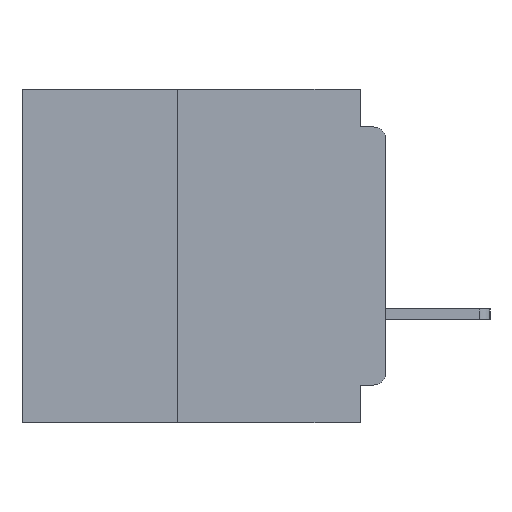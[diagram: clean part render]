
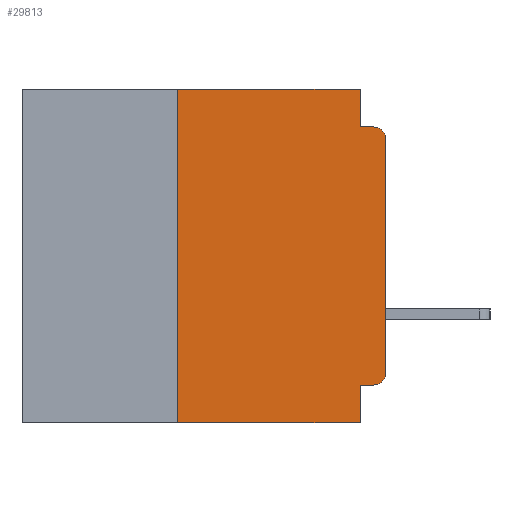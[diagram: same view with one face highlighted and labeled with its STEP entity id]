
A CAD part, left-side view. The second image highlights one B-rep face of the part: STEP entity #29813.
In plain terms, the highlighted planar face has unit normal (-1, 0, 0).
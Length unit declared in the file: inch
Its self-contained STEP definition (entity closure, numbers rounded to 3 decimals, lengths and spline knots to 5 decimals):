
#1818 = ORIENTED_EDGE ( 'NONE', *, *, #26451, .F. ) ;
#2813 = VERTEX_POINT ( 'NONE', #19348 ) ;
#3459 = CARTESIAN_POINT ( 'NONE',  ( 0., 0.031, 0. ) ) ;
#3707 = ORIENTED_EDGE ( 'NONE', *, *, #32260, .T. ) ;
#4417 = DIRECTION ( 'NONE',  ( 0., -1., 0. ) ) ;
#4430 = DIRECTION ( 'NONE',  ( 0., 0., -1. ) ) ;
#5386 = LINE ( 'NONE', #27060, #25469 ) ;
#5630 = DIRECTION ( 'NONE',  ( -1., 0., 0. ) ) ;
#6081 = CARTESIAN_POINT ( 'NONE',  ( 0., 0.25, 0. ) ) ;
#6816 = EDGE_CURVE ( 'NONE', #2813, #23535, #35908, .T. ) ;
#7315 = CARTESIAN_POINT ( 'NONE',  ( 0., 0., -0.355 ) ) ;
#8378 = VECTOR ( 'NONE', #11125, 39.37008 ) ;
#8442 = ORIENTED_EDGE ( 'NONE', *, *, #34644, .F. ) ;
#9361 = EDGE_CURVE ( 'NONE', #30676, #23535, #41780, .T. ) ;
#10786 = CARTESIAN_POINT ( 'NONE',  ( 0., 0.015, -0.06 ) ) ;
#11125 = DIRECTION ( 'NONE',  ( 0., 1., 0. ) ) ;
#11918 = DIRECTION ( 'NONE',  ( 0., -1., 0. ) ) ;
#14106 = LINE ( 'NONE', #39526, #33020 ) ;
#14551 = DIRECTION ( 'NONE',  ( 0., 0., -1. ) ) ;
#15626 = CARTESIAN_POINT ( 'NONE',  ( 0., 0.031, -0.4 ) ) ;
#15832 = AXIS2_PLACEMENT_3D ( 'NONE', #28277, #5630, #32026 ) ;
#17873 = CARTESIAN_POINT ( 'NONE',  ( 0., 0.015, -0.355 ) ) ;
#18451 = ORIENTED_EDGE ( 'NONE', *, *, #46420, .F. ) ;
#18835 = CARTESIAN_POINT ( 'NONE',  ( 0., 0.437, -0.4 ) ) ;
#19348 = CARTESIAN_POINT ( 'NONE',  ( 0., 0.031, -0.355 ) ) ;
#19429 = CARTESIAN_POINT ( 'NONE',  ( 0., 0.437, 0. ) ) ;
#19827 = VERTEX_POINT ( 'NONE', #33638 ) ;
#20649 = LINE ( 'NONE', #33507, #39471 ) ;
#21603 = CARTESIAN_POINT ( 'NONE',  ( 0., 0.031, -0.4 ) ) ;
#21633 = LINE ( 'NONE', #31432, #40445 ) ;
#21799 = AXIS2_PLACEMENT_3D ( 'NONE', #10786, #37174, #14551 ) ;
#23085 = EDGE_CURVE ( 'NONE', #34024, #35416, #23987, .T. ) ;
#23146 = ORIENTED_EDGE ( 'NONE', *, *, #32912, .T. ) ;
#23247 = PLANE ( 'NONE',  #39629 ) ;
#23535 = VERTEX_POINT ( 'NONE', #15626 ) ;
#23712 = VERTEX_POINT ( 'NONE', #6081 ) ;
#23987 = CIRCLE ( 'NONE', #15832, 0.015 ) ;
#24582 = CARTESIAN_POINT ( 'NONE',  ( 0., 0., -0.34 ) ) ;
#24876 = LINE ( 'NONE', #32584, #43674 ) ;
#25469 = VECTOR ( 'NONE', #4417, 39.37008 ) ;
#26451 = EDGE_CURVE ( 'NONE', #23712, #28197, #5386, .T. ) ;
#26641 = ORIENTED_EDGE ( 'NONE', *, *, #6816, .F. ) ;
#27060 = CARTESIAN_POINT ( 'NONE',  ( 0., 0.437, 0. ) ) ;
#27070 = DIRECTION ( 'NONE',  ( 1., 0., 0. ) ) ;
#28197 = VERTEX_POINT ( 'NONE', #3459 ) ;
#28277 = CARTESIAN_POINT ( 'NONE',  ( 0., 0.015, -0.34 ) ) ;
#28514 = LINE ( 'NONE', #7315, #8378 ) ;
#29122 = ORIENTED_EDGE ( 'NONE', *, *, #23085, .T. ) ;
#29813 = ADVANCED_FACE ( 'NONE', ( #33377 ), #23247, .F. ) ;
#29993 = VERTEX_POINT ( 'NONE', #39327 ) ;
#30676 = VERTEX_POINT ( 'NONE', #32399 ) ;
#31432 = CARTESIAN_POINT ( 'NONE',  ( 0., 0.031, 0. ) ) ;
#31828 = VECTOR ( 'NONE', #11918, 39.37008 ) ;
#32026 = DIRECTION ( 'NONE',  ( 0., 0., -1. ) ) ;
#32123 = EDGE_CURVE ( 'NONE', #30676, #23712, #24876, .T. ) ;
#32147 = ORIENTED_EDGE ( 'NONE', *, *, #44845, .F. ) ;
#32260 = EDGE_CURVE ( 'NONE', #40333, #29993, #47748, .T. ) ;
#32399 = CARTESIAN_POINT ( 'NONE',  ( 0., 0.25, -0.4 ) ) ;
#32584 = CARTESIAN_POINT ( 'NONE',  ( 0., 0.25, -0.4 ) ) ;
#32912 = EDGE_CURVE ( 'NONE', #35416, #40333, #20649, .T. ) ;
#33020 = VECTOR ( 'NONE', #43297, 39.37008 ) ;
#33377 = FACE_OUTER_BOUND ( 'NONE', #43327, .T. ) ;
#33507 = CARTESIAN_POINT ( 'NONE',  ( 0., 0., 0. ) ) ;
#33538 = ORIENTED_EDGE ( 'NONE', *, *, #32123, .F. ) ;
#33638 = CARTESIAN_POINT ( 'NONE',  ( 0., 0.031, -0.045 ) ) ;
#34024 = VERTEX_POINT ( 'NONE', #17873 ) ;
#34547 = ORIENTED_EDGE ( 'NONE', *, *, #9361, .T. ) ;
#34644 = EDGE_CURVE ( 'NONE', #28197, #19827, #21633, .T. ) ;
#34742 = VECTOR ( 'NONE', #44118, 39.37008 ) ;
#35186 = DIRECTION ( 'NONE',  ( 0., 0., -1. ) ) ;
#35416 = VERTEX_POINT ( 'NONE', #24582 ) ;
#35908 = LINE ( 'NONE', #21603, #34742 ) ;
#36346 = DIRECTION ( 'NONE',  ( 0., 0., 1. ) ) ;
#36391 = CARTESIAN_POINT ( 'NONE',  ( 0., 0., -0.06 ) ) ;
#37174 = DIRECTION ( 'NONE',  ( -1., 0., 0. ) ) ;
#37276 = DIRECTION ( 'NONE',  ( 0., 0., 1. ) ) ;
#39327 = CARTESIAN_POINT ( 'NONE',  ( 0., 0.015, -0.045 ) ) ;
#39471 = VECTOR ( 'NONE', #37276, 39.37008 ) ;
#39526 = CARTESIAN_POINT ( 'NONE',  ( 0., 0., -0.045 ) ) ;
#39629 = AXIS2_PLACEMENT_3D ( 'NONE', #19429, #27070, #4430 ) ;
#40333 = VERTEX_POINT ( 'NONE', #36391 ) ;
#40445 = VECTOR ( 'NONE', #35186, 39.37008 ) ;
#41780 = LINE ( 'NONE', #18835, #31828 ) ;
#43297 = DIRECTION ( 'NONE',  ( 0., -1., 0. ) ) ;
#43327 = EDGE_LOOP ( 'NONE', ( #23146, #3707, #18451, #8442, #1818, #33538, #34547, #26641, #32147, #29122 ) ) ;
#43674 = VECTOR ( 'NONE', #36346, 39.37008 ) ;
#44118 = DIRECTION ( 'NONE',  ( 0., 0., -1. ) ) ;
#44845 = EDGE_CURVE ( 'NONE', #34024, #2813, #28514, .T. ) ;
#46420 = EDGE_CURVE ( 'NONE', #19827, #29993, #14106, .T. ) ;
#47748 = CIRCLE ( 'NONE', #21799, 0.015 ) ;
